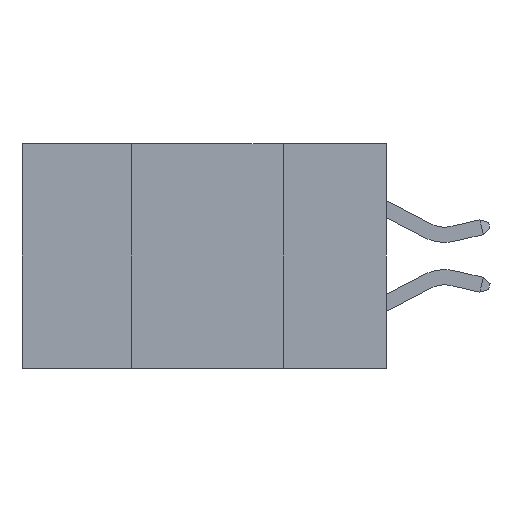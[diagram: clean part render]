
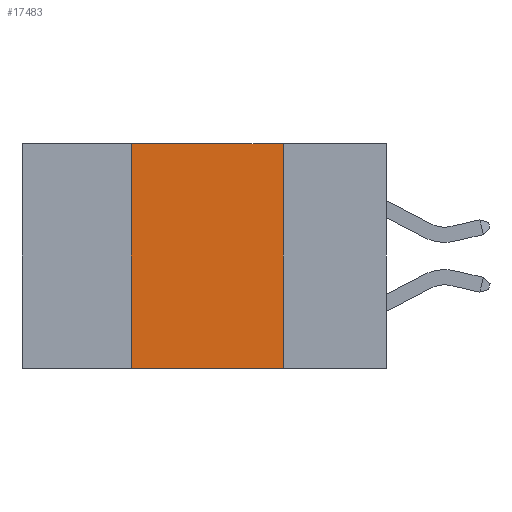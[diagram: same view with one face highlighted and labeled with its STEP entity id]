
A CAD part, left-side view. The second image highlights one B-rep face of the part: STEP entity #17483.
In plain terms, the highlighted planar face has unit normal (-1, 0, 0).
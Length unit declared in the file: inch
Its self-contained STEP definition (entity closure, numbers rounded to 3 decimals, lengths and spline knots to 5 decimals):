
#404 = VERTEX_POINT ( 'NONE', #24361 ) ;
#1396 = VECTOR ( 'NONE', #28149, 39.37008 ) ;
#1739 = AXIS2_PLACEMENT_3D ( 'NONE', #18878, #21478, #26686 ) ;
#2906 = DIRECTION ( 'NONE',  ( 0., -1., 0. ) ) ;
#4452 = ORIENTED_EDGE ( 'NONE', *, *, #28646, .F. ) ;
#5228 = VECTOR ( 'NONE', #2906, 39.37008 ) ;
#5606 = CARTESIAN_POINT ( 'NONE',  ( 0., 0.42, -0.37 ) ) ;
#6319 = ORIENTED_EDGE ( 'NONE', *, *, #33037, .F. ) ;
#8659 = VERTEX_POINT ( 'NONE', #10905 ) ;
#9114 = VERTEX_POINT ( 'NONE', #5606 ) ;
#9707 = EDGE_LOOP ( 'NONE', ( #18881, #4452, #6319, #12256 ) ) ;
#10905 = CARTESIAN_POINT ( 'NONE',  ( 0., 0.17, 0. ) ) ;
#12256 = ORIENTED_EDGE ( 'NONE', *, *, #16580, .T. ) ;
#15173 = LINE ( 'NONE', #29674, #1396 ) ;
#15499 = CARTESIAN_POINT ( 'NONE',  ( 0., 0.42, 0. ) ) ;
#16505 = PLANE ( 'NONE',  #1739 ) ;
#16580 = EDGE_CURVE ( 'NONE', #9114, #404, #25135, .T. ) ;
#16596 = CARTESIAN_POINT ( 'NONE',  ( 0., 0.6, -0.37 ) ) ;
#16939 = DIRECTION ( 'NONE',  ( 0., -1., 0. ) ) ;
#17483 = ADVANCED_FACE ( 'NONE', ( #31954 ), #16505, .F. ) ;
#18332 = CARTESIAN_POINT ( 'NONE',  ( 0., 0.6, 0. ) ) ;
#18878 = CARTESIAN_POINT ( 'NONE',  ( 0., 0.6, 0. ) ) ;
#18881 = ORIENTED_EDGE ( 'NONE', *, *, #24059, .F. ) ;
#21478 = DIRECTION ( 'NONE',  ( 1., 0., 0. ) ) ;
#24059 = EDGE_CURVE ( 'NONE', #8659, #404, #15173, .T. ) ;
#24361 = CARTESIAN_POINT ( 'NONE',  ( 0., 0.17, -0.37 ) ) ;
#25135 = LINE ( 'NONE', #16596, #31203 ) ;
#25208 = VERTEX_POINT ( 'NONE', #28222 ) ;
#26128 = DIRECTION ( 'NONE',  ( 0., 0., 1. ) ) ;
#26404 = VECTOR ( 'NONE', #26128, 39.37008 ) ;
#26686 = DIRECTION ( 'NONE',  ( 0., 0., -1. ) ) ;
#27516 = LINE ( 'NONE', #18332, #5228 ) ;
#28149 = DIRECTION ( 'NONE',  ( 0., 0., -1. ) ) ;
#28222 = CARTESIAN_POINT ( 'NONE',  ( 0., 0.42, 0. ) ) ;
#28646 = EDGE_CURVE ( 'NONE', #25208, #8659, #27516, .T. ) ;
#29674 = CARTESIAN_POINT ( 'NONE',  ( 0., 0.17, 0. ) ) ;
#30499 = LINE ( 'NONE', #15499, #26404 ) ;
#31203 = VECTOR ( 'NONE', #16939, 39.37008 ) ;
#31954 = FACE_OUTER_BOUND ( 'NONE', #9707, .T. ) ;
#33037 = EDGE_CURVE ( 'NONE', #9114, #25208, #30499, .T. ) ;
